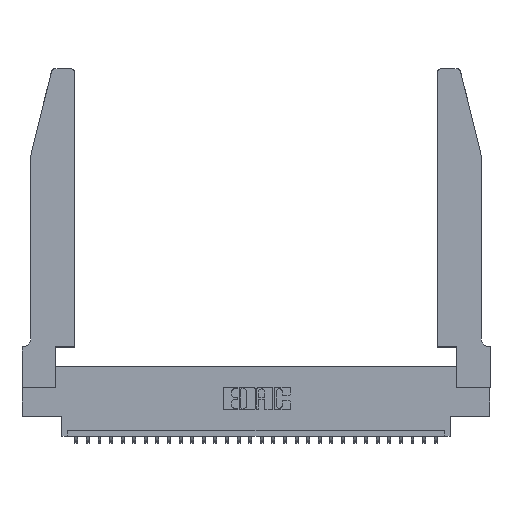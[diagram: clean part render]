
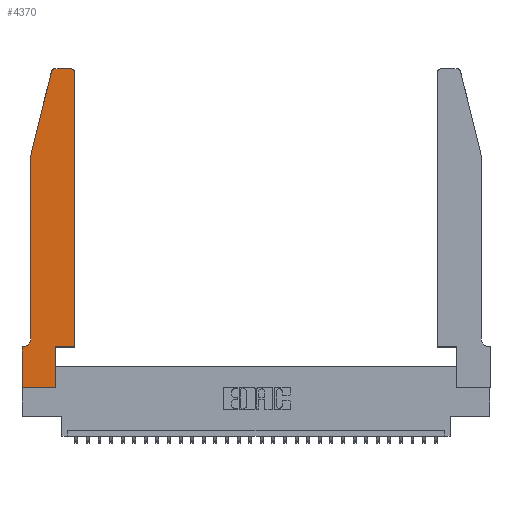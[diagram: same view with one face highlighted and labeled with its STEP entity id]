
A CAD part, top view. The second image highlights one B-rep face of the part: STEP entity #4370.
In plain terms, the highlighted planar face has unit normal (0, 0, 1).
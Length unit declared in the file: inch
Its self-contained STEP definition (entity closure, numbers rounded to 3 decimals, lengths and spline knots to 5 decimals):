
#134 = DIRECTION ( 'NONE',  ( 0., 0., -1. ) ) ;
#495 = DIRECTION ( 'NONE',  ( 1., 0., 0. ) ) ;
#507 = AXIS2_PLACEMENT_3D ( 'NONE', #17887, #10896, #29758 ) ;
#1592 = VECTOR ( 'NONE', #28904, 39.37008 ) ;
#1850 = CARTESIAN_POINT ( 'NONE',  ( 0.25487, 2.72718, 0.37 ) ) ;
#2053 = DIRECTION ( 'NONE',  ( 1., 0., 0. ) ) ;
#2080 = DIRECTION ( 'NONE',  ( 0., 1., 0. ) ) ;
#2309 = DIRECTION ( 'NONE',  ( -1., 0., 0. ) ) ;
#2470 = EDGE_CURVE ( 'NONE', #10413, #15823, #28037, .T. ) ;
#2538 = VECTOR ( 'NONE', #27380, 39.37008 ) ;
#2656 = CARTESIAN_POINT ( 'NONE',  ( 0., 0., 0.37 ) ) ;
#2970 = CARTESIAN_POINT ( 'NONE',  ( 0.284, 2.75, 0.37 ) ) ;
#3956 = EDGE_CURVE ( 'NONE', #14105, #17657, #8554, .T. ) ;
#4254 = CARTESIAN_POINT ( 'NONE',  ( 0.0755, 0.35, 0.37 ) ) ;
#4370 = ADVANCED_FACE ( 'NONE', ( #6004 ), #21691, .T. ) ;
#4517 = CIRCLE ( 'NONE', #16115, 0.07 ) ;
#4586 = DIRECTION ( 'NONE',  ( -1., 0., 0. ) ) ;
#4772 = VECTOR ( 'NONE', #2053, 39.37008 ) ;
#5344 = VECTOR ( 'NONE', #2309, 39.37008 ) ;
#5895 = CARTESIAN_POINT ( 'NONE',  ( 0.4505, 0.35, 0.37 ) ) ;
#6004 = FACE_OUTER_BOUND ( 'NONE', #16553, .T. ) ;
#7095 = VERTEX_POINT ( 'NONE', #21352 ) ;
#7540 = EDGE_CURVE ( 'NONE', #17657, #7095, #14753, .T. ) ;
#7602 = VERTEX_POINT ( 'NONE', #28234 ) ;
#8177 = VERTEX_POINT ( 'NONE', #2656 ) ;
#8554 = CIRCLE ( 'NONE', #30017, 0.03 ) ;
#8930 = CARTESIAN_POINT ( 'NONE',  ( 0.4505, 2.72, 0.37 ) ) ;
#9114 = LINE ( 'NONE', #4254, #14283 ) ;
#10049 = CARTESIAN_POINT ( 'NONE',  ( 0., 0.35, 0.37 ) ) ;
#10351 = LINE ( 'NONE', #25757, #19129 ) ;
#10412 = LINE ( 'NONE', #19665, #1592 ) ;
#10413 = VERTEX_POINT ( 'NONE', #8930 ) ;
#10896 = DIRECTION ( 'NONE',  ( 0., 0., 1. ) ) ;
#11048 = CARTESIAN_POINT ( 'NONE',  ( 0.2865, 0.35, 0.37 ) ) ;
#11308 = LINE ( 'NONE', #25842, #4772 ) ;
#11408 = ORIENTED_EDGE ( 'NONE', *, *, #23982, .T. ) ;
#11430 = VECTOR ( 'NONE', #13625, 39.37008 ) ;
#12698 = VERTEX_POINT ( 'NONE', #26259 ) ;
#12791 = ORIENTED_EDGE ( 'NONE', *, *, #23887, .T. ) ;
#13085 = EDGE_CURVE ( 'NONE', #23562, #10413, #20091, .T. ) ;
#13334 = ORIENTED_EDGE ( 'NONE', *, *, #13085, .T. ) ;
#13575 = ORIENTED_EDGE ( 'NONE', *, *, #15804, .T. ) ;
#13625 = DIRECTION ( 'NONE',  ( -0.239, -0.971, 0. ) ) ;
#13627 = CARTESIAN_POINT ( 'NONE',  ( 0.0755, 2., 0.37 ) ) ;
#14105 = VERTEX_POINT ( 'NONE', #2970 ) ;
#14150 = CARTESIAN_POINT ( 'NONE',  ( 0., 0.35, 0.37 ) ) ;
#14283 = VECTOR ( 'NONE', #25326, 39.37008 ) ;
#14753 = LINE ( 'NONE', #27453, #11430 ) ;
#15804 = EDGE_CURVE ( 'NONE', #18534, #23562, #10412, .T. ) ;
#15823 = VERTEX_POINT ( 'NONE', #26628 ) ;
#15865 = CARTESIAN_POINT ( 'NONE',  ( 0.2865, 0., 0.37 ) ) ;
#16115 = AXIS2_PLACEMENT_3D ( 'NONE', #16255, #134, #4586 ) ;
#16255 = CARTESIAN_POINT ( 'NONE',  ( 0.0055, 0.42, 0.37 ) ) ;
#16553 = EDGE_LOOP ( 'NONE', ( #28453, #17119, #24320, #27368, #17031, #11408, #12791, #17073, #25996, #13575, #13334, #20426 ) ) ;
#16668 = DIRECTION ( 'NONE',  ( 1., 0., 0. ) ) ;
#16696 = EDGE_CURVE ( 'NONE', #7602, #12698, #4517, .T. ) ;
#16765 = CARTESIAN_POINT ( 'NONE',  ( 0.284, 2.72, 0.37 ) ) ;
#16961 = EDGE_CURVE ( 'NONE', #26813, #18534, #10351, .T. ) ;
#17031 = ORIENTED_EDGE ( 'NONE', *, *, #16696, .T. ) ;
#17073 = ORIENTED_EDGE ( 'NONE', *, *, #24125, .T. ) ;
#17119 = ORIENTED_EDGE ( 'NONE', *, *, #3956, .T. ) ;
#17657 = VERTEX_POINT ( 'NONE', #1850 ) ;
#17887 = CARTESIAN_POINT ( 'NONE',  ( 0.4205, 2.72, 0.37 ) ) ;
#18432 = VERTEX_POINT ( 'NONE', #14150 ) ;
#18440 = AXIS2_PLACEMENT_3D ( 'NONE', #10049, #23866, #495 ) ;
#18534 = VERTEX_POINT ( 'NONE', #11048 ) ;
#19129 = VECTOR ( 'NONE', #2080, 39.37008 ) ;
#19665 = CARTESIAN_POINT ( 'NONE',  ( 0.4505, 0.35, 0.37 ) ) ;
#20091 = LINE ( 'NONE', #5895, #21544 ) ;
#20426 = ORIENTED_EDGE ( 'NONE', *, *, #2470, .T. ) ;
#21352 = CARTESIAN_POINT ( 'NONE',  ( 0.0755, 2., 0.37 ) ) ;
#21544 = VECTOR ( 'NONE', #26462, 39.37008 ) ;
#21691 = PLANE ( 'NONE',  #18440 ) ;
#22549 = VECTOR ( 'NONE', #30118, 39.37008 ) ;
#23030 = LINE ( 'NONE', #25025, #2538 ) ;
#23562 = VERTEX_POINT ( 'NONE', #28619 ) ;
#23866 = DIRECTION ( 'NONE',  ( 0., 0., 1. ) ) ;
#23887 = EDGE_CURVE ( 'NONE', #18432, #8177, #23030, .T. ) ;
#23982 = EDGE_CURVE ( 'NONE', #12698, #18432, #9114, .T. ) ;
#24125 = EDGE_CURVE ( 'NONE', #8177, #26813, #11308, .T. ) ;
#24320 = ORIENTED_EDGE ( 'NONE', *, *, #7540, .T. ) ;
#25025 = CARTESIAN_POINT ( 'NONE',  ( 0., 0., 0.37 ) ) ;
#25326 = DIRECTION ( 'NONE',  ( -1., 0., 0. ) ) ;
#25757 = CARTESIAN_POINT ( 'NONE',  ( 0.2865, 0.35, 0.37 ) ) ;
#25842 = CARTESIAN_POINT ( 'NONE',  ( 0., 0., 0.37 ) ) ;
#25996 = ORIENTED_EDGE ( 'NONE', *, *, #16961, .T. ) ;
#26259 = CARTESIAN_POINT ( 'NONE',  ( 0.0055, 0.35, 0.37 ) ) ;
#26462 = DIRECTION ( 'NONE',  ( 0., 1., 0. ) ) ;
#26573 = EDGE_CURVE ( 'NONE', #7095, #7602, #27322, .T. ) ;
#26628 = CARTESIAN_POINT ( 'NONE',  ( 0.4205, 2.75, 0.37 ) ) ;
#26813 = VERTEX_POINT ( 'NONE', #15865 ) ;
#26952 = EDGE_CURVE ( 'NONE', #15823, #14105, #30257, .T. ) ;
#27322 = LINE ( 'NONE', #13627, #22549 ) ;
#27368 = ORIENTED_EDGE ( 'NONE', *, *, #26573, .T. ) ;
#27380 = DIRECTION ( 'NONE',  ( 0., -1., 0. ) ) ;
#27453 = CARTESIAN_POINT ( 'NONE',  ( 0.0755, 2., 0.37 ) ) ;
#28037 = CIRCLE ( 'NONE', #507, 0.03 ) ;
#28109 = DIRECTION ( 'NONE',  ( 0., 0., 1. ) ) ;
#28234 = CARTESIAN_POINT ( 'NONE',  ( 0.0755, 0.42, 0.37 ) ) ;
#28453 = ORIENTED_EDGE ( 'NONE', *, *, #26952, .T. ) ;
#28619 = CARTESIAN_POINT ( 'NONE',  ( 0.4505, 0.35, 0.37 ) ) ;
#28904 = DIRECTION ( 'NONE',  ( 1., 0., 0. ) ) ;
#29758 = DIRECTION ( 'NONE',  ( 1., 0., 0. ) ) ;
#30017 = AXIS2_PLACEMENT_3D ( 'NONE', #16765, #28109, #16668 ) ;
#30118 = DIRECTION ( 'NONE',  ( 0., -1., 0. ) ) ;
#30257 = LINE ( 'NONE', #30409, #5344 ) ;
#30409 = CARTESIAN_POINT ( 'NONE',  ( 0.2605, 2.75, 0.37 ) ) ;
